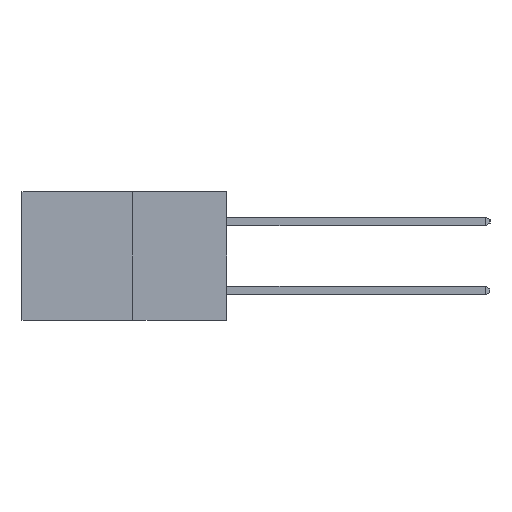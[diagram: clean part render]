
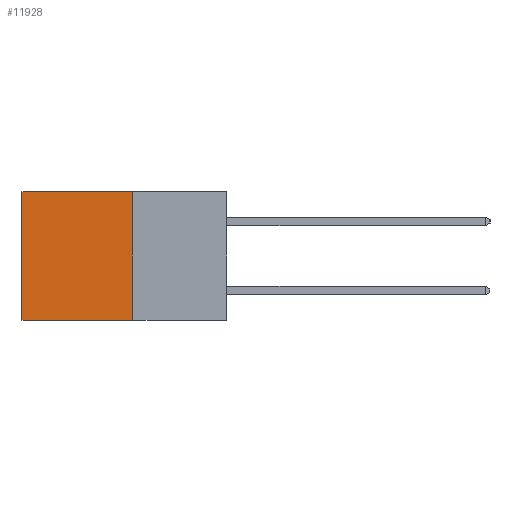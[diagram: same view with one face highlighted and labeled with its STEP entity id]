
A CAD part, left-side view. The second image highlights one B-rep face of the part: STEP entity #11928.
In plain terms, the highlighted planar face has unit normal (-1, 0, 0).
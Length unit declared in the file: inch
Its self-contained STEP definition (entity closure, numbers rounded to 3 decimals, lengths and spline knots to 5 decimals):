
#164 = ORIENTED_EDGE ( 'NONE', *, *, #7746, .F. ) ;
#193 = VECTOR ( 'NONE', #7608, 39.37008 ) ;
#336 = CARTESIAN_POINT ( 'NONE',  ( 0.277, 0.27, -0.37 ) ) ;
#759 = VECTOR ( 'NONE', #7506, 39.37008 ) ;
#1312 = EDGE_CURVE ( 'NONE', #1756, #11511, #10620, .T. ) ;
#1756 = VERTEX_POINT ( 'NONE', #8008 ) ;
#2421 = EDGE_CURVE ( 'NONE', #5110, #11511, #10746, .T. ) ;
#2535 = DIRECTION ( 'NONE',  ( 0., 0., -1. ) ) ;
#2685 = CARTESIAN_POINT ( 'NONE',  ( 0.277, 0.27, 0. ) ) ;
#2762 = DIRECTION ( 'NONE',  ( 1., 0., 0. ) ) ;
#3416 = AXIS2_PLACEMENT_3D ( 'NONE', #8843, #2762, #9841 ) ;
#3630 = EDGE_LOOP ( 'NONE', ( #6321, #9971, #164, #8883 ) ) ;
#4306 = VERTEX_POINT ( 'NONE', #2685 ) ;
#5110 = VERTEX_POINT ( 'NONE', #336 ) ;
#5551 = LINE ( 'NONE', #12531, #193 ) ;
#5667 = VECTOR ( 'NONE', #9218, 39.37008 ) ;
#6321 = ORIENTED_EDGE ( 'NONE', *, *, #1312, .T. ) ;
#7506 = DIRECTION ( 'NONE',  ( 0., 0., -1. ) ) ;
#7608 = DIRECTION ( 'NONE',  ( 0., 1., 0. ) ) ;
#7746 = EDGE_CURVE ( 'NONE', #4306, #5110, #8853, .T. ) ;
#7823 = PLANE ( 'NONE',  #3416 ) ;
#8008 = CARTESIAN_POINT ( 'NONE',  ( 0.277, 0.59, 0. ) ) ;
#8843 = CARTESIAN_POINT ( 'NONE',  ( 0.277, 0.27, -0.37 ) ) ;
#8853 = LINE ( 'NONE', #12444, #759 ) ;
#8883 = ORIENTED_EDGE ( 'NONE', *, *, #11811, .T. ) ;
#9061 = CARTESIAN_POINT ( 'NONE',  ( 0.277, 0.27, -0.37 ) ) ;
#9218 = DIRECTION ( 'NONE',  ( 0., 1., 0. ) ) ;
#9841 = DIRECTION ( 'NONE',  ( 0., 0., -1. ) ) ;
#9971 = ORIENTED_EDGE ( 'NONE', *, *, #2421, .F. ) ;
#10214 = CARTESIAN_POINT ( 'NONE',  ( 0.277, 0.59, -0.37 ) ) ;
#10620 = LINE ( 'NONE', #11749, #12576 ) ;
#10746 = LINE ( 'NONE', #9061, #5667 ) ;
#11384 = FACE_OUTER_BOUND ( 'NONE', #3630, .T. ) ;
#11511 = VERTEX_POINT ( 'NONE', #10214 ) ;
#11749 = CARTESIAN_POINT ( 'NONE',  ( 0.277, 0.59, -0.37 ) ) ;
#11811 = EDGE_CURVE ( 'NONE', #4306, #1756, #5551, .T. ) ;
#11928 = ADVANCED_FACE ( 'NONE', ( #11384 ), #7823, .F. ) ;
#12444 = CARTESIAN_POINT ( 'NONE',  ( 0.277, 0.27, -0.37 ) ) ;
#12531 = CARTESIAN_POINT ( 'NONE',  ( 0.277, 0.27, 0. ) ) ;
#12576 = VECTOR ( 'NONE', #2535, 39.37008 ) ;
